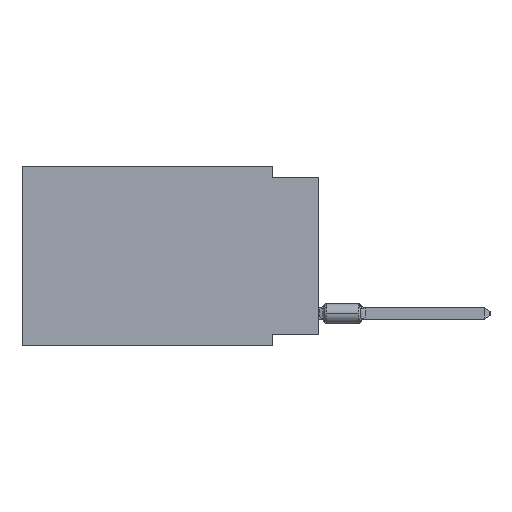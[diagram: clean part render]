
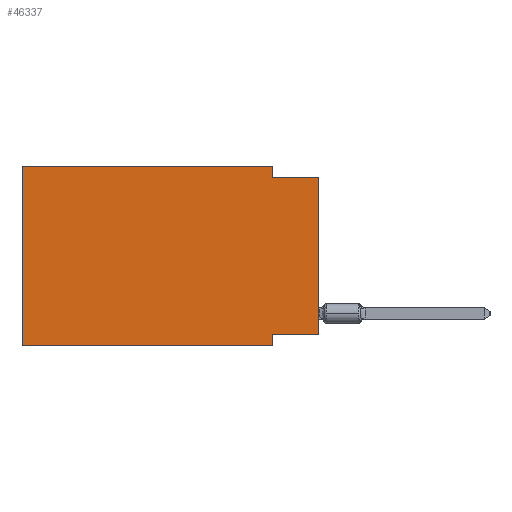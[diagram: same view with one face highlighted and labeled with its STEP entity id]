
A CAD part, left-side view. The second image highlights one B-rep face of the part: STEP entity #46337.
In plain terms, the highlighted planar face has unit normal (-1, 0, 0).
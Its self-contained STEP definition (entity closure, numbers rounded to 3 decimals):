
#417 = AXIS2_PLACEMENT_3D ( 'NONE', #6042, #21113, #26350 ) ;
#724 = VERTEX_POINT ( 'NONE', #6832 ) ;
#1582 = ORIENTED_EDGE ( 'NONE', *, *, #9383, .T. ) ;
#1649 = CARTESIAN_POINT ( 'NONE',  ( 0., 2.54, -9.906 ) ) ;
#1662 = CARTESIAN_POINT ( 'NONE',  ( 0., 0., -9.271 ) ) ;
#4476 = DIRECTION ( 'NONE',  ( 0., -1., 0. ) ) ;
#4525 = CARTESIAN_POINT ( 'NONE',  ( 0., 2.54, 0. ) ) ;
#5500 = DIRECTION ( 'NONE',  ( 0., 0., -1. ) ) ;
#6042 = CARTESIAN_POINT ( 'NONE',  ( 0., 16.383, 0. ) ) ;
#6309 = VECTOR ( 'NONE', #56411, 1000. ) ;
#6743 = DIRECTION ( 'NONE',  ( 0., -1., 0. ) ) ;
#6832 = CARTESIAN_POINT ( 'NONE',  ( 0., 0., -0.635 ) ) ;
#7214 = LINE ( 'NONE', #17690, #6309 ) ;
#8605 = VECTOR ( 'NONE', #60063, 1000. ) ;
#9383 = EDGE_CURVE ( 'NONE', #43475, #724, #34508, .T. ) ;
#11613 = VECTOR ( 'NONE', #4476, 1000. ) ;
#11967 = CARTESIAN_POINT ( 'NONE',  ( 0., 16.383, -9.906 ) ) ;
#12204 = ORIENTED_EDGE ( 'NONE', *, *, #61181, .T. ) ;
#13164 = VECTOR ( 'NONE', #6743, 1000. ) ;
#14598 = CARTESIAN_POINT ( 'NONE',  ( 0., 0., -9.271 ) ) ;
#15151 = CARTESIAN_POINT ( 'NONE',  ( 0., 0., 0. ) ) ;
#16520 = FACE_OUTER_BOUND ( 'NONE', #35918, .T. ) ;
#16732 = LINE ( 'NONE', #1649, #60779 ) ;
#17690 = CARTESIAN_POINT ( 'NONE',  ( 0., 16.383, 0. ) ) ;
#18682 = ORIENTED_EDGE ( 'NONE', *, *, #57816, .F. ) ;
#21113 = DIRECTION ( 'NONE',  ( 1., 0., 0. ) ) ;
#21639 = DIRECTION ( 'NONE',  ( 0., 0., -1. ) ) ;
#22356 = VERTEX_POINT ( 'NONE', #54490 ) ;
#22754 = EDGE_CURVE ( 'NONE', #33947, #29944, #59901, .T. ) ;
#23157 = LINE ( 'NONE', #48090, #11613 ) ;
#24466 = VECTOR ( 'NONE', #24812, 1000. ) ;
#24812 = DIRECTION ( 'NONE',  ( 0., 0., 1. ) ) ;
#25303 = CARTESIAN_POINT ( 'NONE',  ( 0., 2.54, -0.635 ) ) ;
#26350 = DIRECTION ( 'NONE',  ( 0., 0., -1. ) ) ;
#29040 = ORIENTED_EDGE ( 'NONE', *, *, #42234, .F. ) ;
#29275 = ORIENTED_EDGE ( 'NONE', *, *, #22754, .F. ) ;
#29944 = VERTEX_POINT ( 'NONE', #33946 ) ;
#29995 = EDGE_CURVE ( 'NONE', #43475, #40674, #63784, .T. ) ;
#33946 = CARTESIAN_POINT ( 'NONE',  ( 0., 16.383, 0. ) ) ;
#33947 = VERTEX_POINT ( 'NONE', #56654 ) ;
#34508 = LINE ( 'NONE', #15151, #8605 ) ;
#35918 = EDGE_LOOP ( 'NONE', ( #1582, #18682, #50109, #29040, #29275, #12204, #38267, #57607 ) ) ;
#36460 = VECTOR ( 'NONE', #38525, 1000. ) ;
#38267 = ORIENTED_EDGE ( 'NONE', *, *, #42306, .F. ) ;
#38525 = DIRECTION ( 'NONE',  ( 0., 1., 0. ) ) ;
#40674 = VERTEX_POINT ( 'NONE', #63289 ) ;
#40815 = CARTESIAN_POINT ( 'NONE',  ( 0., 2.54, -9.906 ) ) ;
#41487 = LINE ( 'NONE', #11967, #13164 ) ;
#42234 = EDGE_CURVE ( 'NONE', #29944, #22356, #7214, .T. ) ;
#42306 = EDGE_CURVE ( 'NONE', #40674, #48018, #16732, .T. ) ;
#43475 = VERTEX_POINT ( 'NONE', #1662 ) ;
#45487 = LINE ( 'NONE', #4525, #54087 ) ;
#46337 = ADVANCED_FACE ( 'NONE', ( #16520 ), #60797, .F. ) ;
#46637 = VERTEX_POINT ( 'NONE', #25303 ) ;
#48018 = VERTEX_POINT ( 'NONE', #40815 ) ;
#48090 = CARTESIAN_POINT ( 'NONE',  ( 0., 0., -0.635 ) ) ;
#49419 = CARTESIAN_POINT ( 'NONE',  ( 0., 16.383, 0. ) ) ;
#50109 = ORIENTED_EDGE ( 'NONE', *, *, #63441, .F. ) ;
#54087 = VECTOR ( 'NONE', #5500, 1000. ) ;
#54490 = CARTESIAN_POINT ( 'NONE',  ( 0., 2.54, 0. ) ) ;
#56411 = DIRECTION ( 'NONE',  ( 0., -1., 0. ) ) ;
#56654 = CARTESIAN_POINT ( 'NONE',  ( 0., 16.383, -9.906 ) ) ;
#57607 = ORIENTED_EDGE ( 'NONE', *, *, #29995, .F. ) ;
#57816 = EDGE_CURVE ( 'NONE', #46637, #724, #23157, .T. ) ;
#59901 = LINE ( 'NONE', #49419, #24466 ) ;
#60063 = DIRECTION ( 'NONE',  ( 0., 0., 1. ) ) ;
#60779 = VECTOR ( 'NONE', #21639, 1000. ) ;
#60797 = PLANE ( 'NONE',  #417 ) ;
#61181 = EDGE_CURVE ( 'NONE', #33947, #48018, #41487, .T. ) ;
#63289 = CARTESIAN_POINT ( 'NONE',  ( 0., 2.54, -9.271 ) ) ;
#63441 = EDGE_CURVE ( 'NONE', #22356, #46637, #45487, .T. ) ;
#63784 = LINE ( 'NONE', #14598, #36460 ) ;
